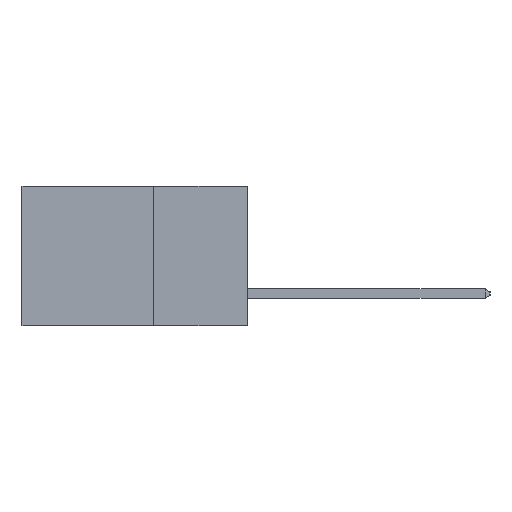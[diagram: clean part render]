
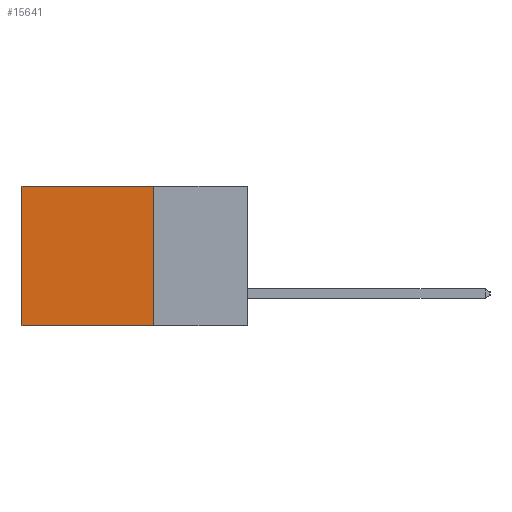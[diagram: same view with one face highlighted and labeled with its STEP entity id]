
A CAD part, left-side view. The second image highlights one B-rep face of the part: STEP entity #15641.
In plain terms, the highlighted planar face has unit normal (-1, 0, 0).
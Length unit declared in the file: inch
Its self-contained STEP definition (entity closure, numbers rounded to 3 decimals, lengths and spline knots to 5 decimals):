
#45 = CARTESIAN_POINT ( 'NONE',  ( 0.2615, 0.25, 0. ) ) ;
#422 = PLANE ( 'NONE',  #7898 ) ;
#479 = DIRECTION ( 'NONE',  ( 1., 0., 0. ) ) ;
#480 = EDGE_CURVE ( 'NONE', #3565, #14517, #14686, .T. ) ;
#1256 = EDGE_CURVE ( 'NONE', #14517, #9399, #1976, .T. ) ;
#1439 = CARTESIAN_POINT ( 'NONE',  ( 0.2615, 0.25, 0. ) ) ;
#1976 = LINE ( 'NONE', #11248, #15009 ) ;
#2298 = DIRECTION ( 'NONE',  ( 0., 0., -1. ) ) ;
#2819 = DIRECTION ( 'NONE',  ( 0., 1., 0. ) ) ;
#2909 = EDGE_CURVE ( 'NONE', #4144, #9399, #10574, .T. ) ;
#3155 = CARTESIAN_POINT ( 'NONE',  ( 0.2615, 0.25, -0.37 ) ) ;
#3344 = ORIENTED_EDGE ( 'NONE', *, *, #480, .F. ) ;
#3565 = VERTEX_POINT ( 'NONE', #45 ) ;
#3897 = ORIENTED_EDGE ( 'NONE', *, *, #1256, .F. ) ;
#4144 = VERTEX_POINT ( 'NONE', #10395 ) ;
#4799 = CARTESIAN_POINT ( 'NONE',  ( 0.2615, 0.6, -0.37 ) ) ;
#5102 = DIRECTION ( 'NONE',  ( 0., 0., -1. ) ) ;
#5132 = FACE_OUTER_BOUND ( 'NONE', #8899, .T. ) ;
#6975 = CARTESIAN_POINT ( 'NONE',  ( 0.2615, 0.6, -0.37 ) ) ;
#7241 = VECTOR ( 'NONE', #5102, 39.37008 ) ;
#7666 = ORIENTED_EDGE ( 'NONE', *, *, #10039, .T. ) ;
#7898 = AXIS2_PLACEMENT_3D ( 'NONE', #8479, #479, #9744 ) ;
#8170 = LINE ( 'NONE', #1439, #11872 ) ;
#8479 = CARTESIAN_POINT ( 'NONE',  ( 0.2615, 0.25, -0.37 ) ) ;
#8899 = EDGE_LOOP ( 'NONE', ( #13041, #3897, #3344, #7666 ) ) ;
#9399 = VERTEX_POINT ( 'NONE', #6975 ) ;
#9744 = DIRECTION ( 'NONE',  ( 0., 0., -1. ) ) ;
#10039 = EDGE_CURVE ( 'NONE', #3565, #4144, #8170, .T. ) ;
#10395 = CARTESIAN_POINT ( 'NONE',  ( 0.2615, 0.6, 0. ) ) ;
#10574 = LINE ( 'NONE', #4799, #7241 ) ;
#11248 = CARTESIAN_POINT ( 'NONE',  ( 0.2615, 0.25, -0.37 ) ) ;
#11302 = DIRECTION ( 'NONE',  ( 0., 1., 0. ) ) ;
#11463 = VECTOR ( 'NONE', #2298, 39.37008 ) ;
#11872 = VECTOR ( 'NONE', #2819, 39.37008 ) ;
#13041 = ORIENTED_EDGE ( 'NONE', *, *, #2909, .T. ) ;
#14162 = CARTESIAN_POINT ( 'NONE',  ( 0.2615, 0.25, -0.37 ) ) ;
#14517 = VERTEX_POINT ( 'NONE', #14162 ) ;
#14686 = LINE ( 'NONE', #3155, #11463 ) ;
#15009 = VECTOR ( 'NONE', #11302, 39.37008 ) ;
#15641 = ADVANCED_FACE ( 'NONE', ( #5132 ), #422, .F. ) ;
